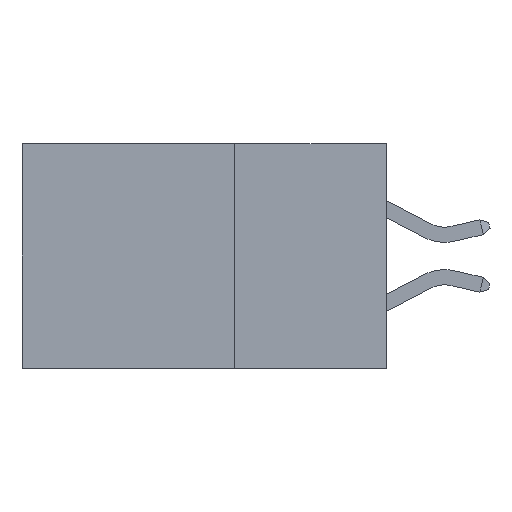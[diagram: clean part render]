
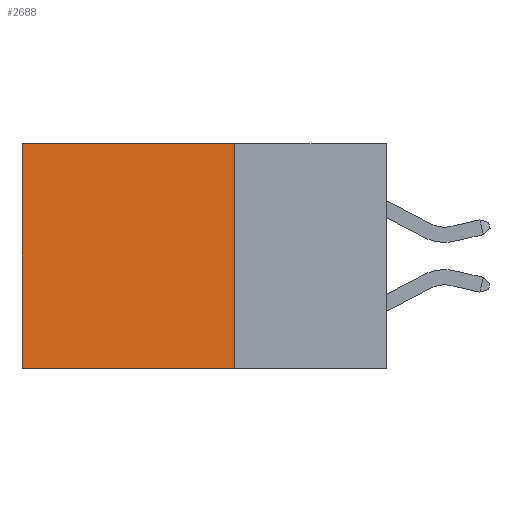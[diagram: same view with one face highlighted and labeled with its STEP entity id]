
A CAD part, left-side view. The second image highlights one B-rep face of the part: STEP entity #2688.
In plain terms, the highlighted planar face has unit normal (-1, 0, 0).
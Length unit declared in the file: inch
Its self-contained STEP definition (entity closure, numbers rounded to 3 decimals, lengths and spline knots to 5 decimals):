
#500 = VECTOR ( 'NONE', #6221, 39.37008 ) ;
#1152 = LINE ( 'NONE', #7003, #14167 ) ;
#2059 = CARTESIAN_POINT ( 'NONE',  ( 0.298, 0.6, -0.37 ) ) ;
#2083 = AXIS2_PLACEMENT_3D ( 'NONE', #9121, #15086, #15072 ) ;
#2142 = VECTOR ( 'NONE', #3258, 39.37008 ) ;
#2688 = ADVANCED_FACE ( 'NONE', ( #7494 ), #14613, .F. ) ;
#3046 = ORIENTED_EDGE ( 'NONE', *, *, #12327, .T. ) ;
#3258 = DIRECTION ( 'NONE',  ( 0., 0., -1. ) ) ;
#4465 = CARTESIAN_POINT ( 'NONE',  ( 0.298, 0.6, 0. ) ) ;
#5011 = CARTESIAN_POINT ( 'NONE',  ( 0.298, 0.25, 0. ) ) ;
#6221 = DIRECTION ( 'NONE',  ( 0., 1., 0. ) ) ;
#6265 = CARTESIAN_POINT ( 'NONE',  ( 0.298, 0.25, -0.37 ) ) ;
#6464 = EDGE_LOOP ( 'NONE', ( #3046, #12537, #9760, #12895 ) ) ;
#7003 = CARTESIAN_POINT ( 'NONE',  ( 0.298, 0.25, 0. ) ) ;
#7235 = LINE ( 'NONE', #5011, #500 ) ;
#7494 = FACE_OUTER_BOUND ( 'NONE', #6464, .T. ) ;
#8092 = CARTESIAN_POINT ( 'NONE',  ( 0.298, 0.25, -0.37 ) ) ;
#8268 = EDGE_CURVE ( 'NONE', #10045, #8521, #1152, .T. ) ;
#8521 = VERTEX_POINT ( 'NONE', #6265 ) ;
#9058 = VERTEX_POINT ( 'NONE', #10860 ) ;
#9121 = CARTESIAN_POINT ( 'NONE',  ( 0.298, 0.25, 0. ) ) ;
#9518 = VERTEX_POINT ( 'NONE', #2059 ) ;
#9760 = ORIENTED_EDGE ( 'NONE', *, *, #8268, .F. ) ;
#10045 = VERTEX_POINT ( 'NONE', #10140 ) ;
#10140 = CARTESIAN_POINT ( 'NONE',  ( 0.298, 0.25, 0. ) ) ;
#10502 = DIRECTION ( 'NONE',  ( 0., 1., 0. ) ) ;
#10685 = EDGE_CURVE ( 'NONE', #10045, #9058, #7235, .T. ) ;
#10778 = VECTOR ( 'NONE', #10502, 39.37008 ) ;
#10860 = CARTESIAN_POINT ( 'NONE',  ( 0.298, 0.6, 0. ) ) ;
#11059 = EDGE_CURVE ( 'NONE', #8521, #9518, #13881, .T. ) ;
#11676 = LINE ( 'NONE', #4465, #2142 ) ;
#12327 = EDGE_CURVE ( 'NONE', #9058, #9518, #11676, .T. ) ;
#12537 = ORIENTED_EDGE ( 'NONE', *, *, #11059, .F. ) ;
#12895 = ORIENTED_EDGE ( 'NONE', *, *, #10685, .T. ) ;
#13881 = LINE ( 'NONE', #8092, #10778 ) ;
#14167 = VECTOR ( 'NONE', #15267, 39.37008 ) ;
#14613 = PLANE ( 'NONE',  #2083 ) ;
#15072 = DIRECTION ( 'NONE',  ( 0., 0., -1. ) ) ;
#15086 = DIRECTION ( 'NONE',  ( 1., 0., 0. ) ) ;
#15267 = DIRECTION ( 'NONE',  ( 0., 0., -1. ) ) ;
